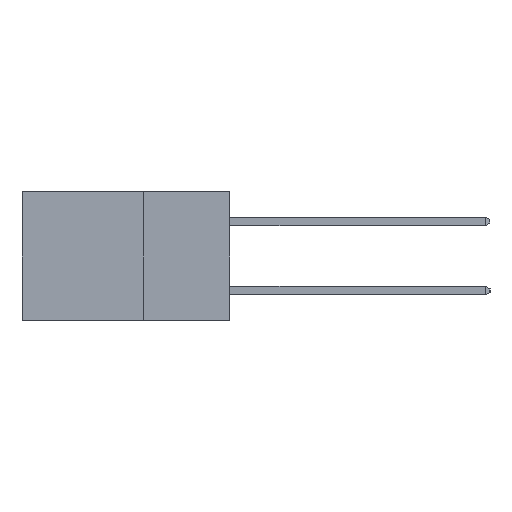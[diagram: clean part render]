
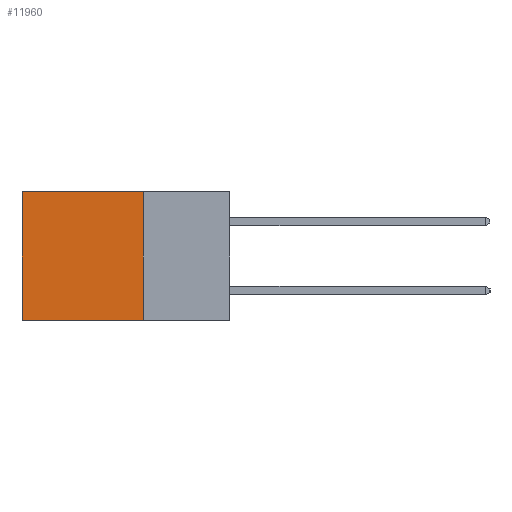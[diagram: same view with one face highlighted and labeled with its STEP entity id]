
A CAD part, left-side view. The second image highlights one B-rep face of the part: STEP entity #11960.
In plain terms, the highlighted planar face has unit normal (-1, 0, 0).
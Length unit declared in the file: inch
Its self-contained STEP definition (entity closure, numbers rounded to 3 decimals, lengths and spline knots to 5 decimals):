
#36 = VECTOR ( 'NONE', #9394, 39.37008 ) ;
#1076 = LINE ( 'NONE', #6727, #11658 ) ;
#1165 = FACE_OUTER_BOUND ( 'NONE', #12409, .T. ) ;
#1348 = DIRECTION ( 'NONE',  ( 0., 1., 0. ) ) ;
#1627 = VECTOR ( 'NONE', #13080, 39.37008 ) ;
#1855 = ORIENTED_EDGE ( 'NONE', *, *, #3212, .T. ) ;
#2740 = VECTOR ( 'NONE', #1348, 39.37008 ) ;
#2866 = CARTESIAN_POINT ( 'NONE',  ( 0.2615, 0.6, 0. ) ) ;
#3036 = CARTESIAN_POINT ( 'NONE',  ( 0.2615, 0.25, 0. ) ) ;
#3092 = EDGE_CURVE ( 'NONE', #5296, #10751, #10159, .T. ) ;
#3212 = EDGE_CURVE ( 'NONE', #12286, #5296, #11288, .T. ) ;
#3910 = AXIS2_PLACEMENT_3D ( 'NONE', #6274, #5951, #5946 ) ;
#4836 = CARTESIAN_POINT ( 'NONE',  ( 0.2615, 0.25, 0. ) ) ;
#4885 = CARTESIAN_POINT ( 'NONE',  ( 0.2615, 0.6, -0.37 ) ) ;
#4926 = VERTEX_POINT ( 'NONE', #12809 ) ;
#5296 = VERTEX_POINT ( 'NONE', #2866 ) ;
#5830 = EDGE_CURVE ( 'NONE', #12286, #4926, #8479, .T. ) ;
#5876 = CARTESIAN_POINT ( 'NONE',  ( 0.2615, 0.6, -0.37 ) ) ;
#5946 = DIRECTION ( 'NONE',  ( 0., 0., -1. ) ) ;
#5951 = DIRECTION ( 'NONE',  ( 1., 0., 0. ) ) ;
#5992 = PLANE ( 'NONE',  #3910 ) ;
#6274 = CARTESIAN_POINT ( 'NONE',  ( 0.2615, 0.25, -0.37 ) ) ;
#6661 = ORIENTED_EDGE ( 'NONE', *, *, #5830, .F. ) ;
#6727 = CARTESIAN_POINT ( 'NONE',  ( 0.2615, 0.25, -0.37 ) ) ;
#6825 = DIRECTION ( 'NONE',  ( 0., 1., 0. ) ) ;
#7086 = ORIENTED_EDGE ( 'NONE', *, *, #3092, .T. ) ;
#8479 = LINE ( 'NONE', #9395, #36 ) ;
#9394 = DIRECTION ( 'NONE',  ( 0., 0., -1. ) ) ;
#9395 = CARTESIAN_POINT ( 'NONE',  ( 0.2615, 0.25, -0.37 ) ) ;
#9568 = EDGE_CURVE ( 'NONE', #4926, #10751, #1076, .T. ) ;
#10159 = LINE ( 'NONE', #4885, #1627 ) ;
#10751 = VERTEX_POINT ( 'NONE', #5876 ) ;
#11288 = LINE ( 'NONE', #3036, #2740 ) ;
#11584 = ORIENTED_EDGE ( 'NONE', *, *, #9568, .F. ) ;
#11658 = VECTOR ( 'NONE', #6825, 39.37008 ) ;
#11960 = ADVANCED_FACE ( 'NONE', ( #1165 ), #5992, .F. ) ;
#12286 = VERTEX_POINT ( 'NONE', #4836 ) ;
#12409 = EDGE_LOOP ( 'NONE', ( #7086, #11584, #6661, #1855 ) ) ;
#12809 = CARTESIAN_POINT ( 'NONE',  ( 0.2615, 0.25, -0.37 ) ) ;
#13080 = DIRECTION ( 'NONE',  ( 0., 0., -1. ) ) ;
